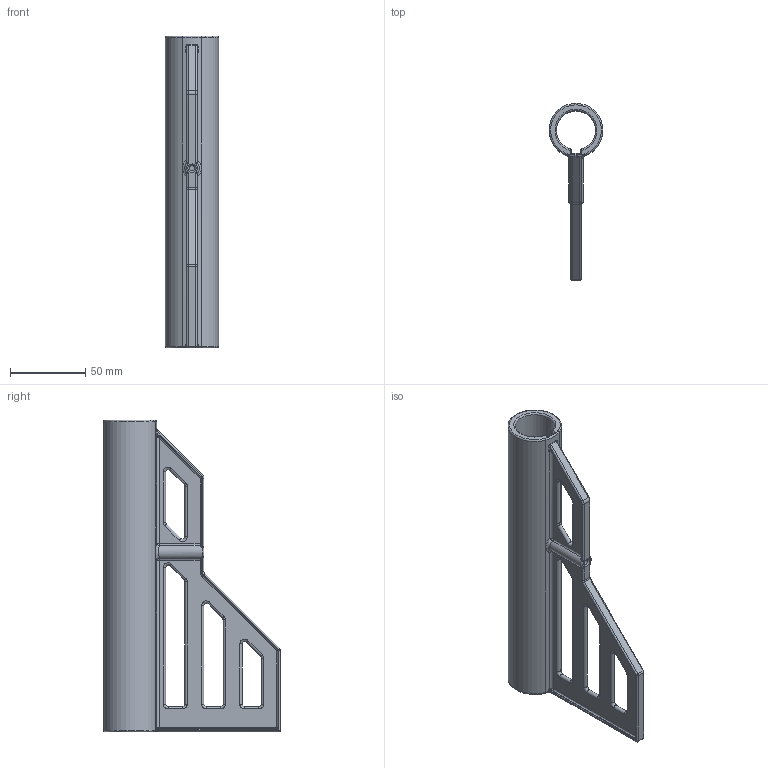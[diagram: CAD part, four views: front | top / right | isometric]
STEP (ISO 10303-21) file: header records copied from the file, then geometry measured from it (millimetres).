
FILE_DESCRIPTION(/* description */ (''),/* implementation_level */ '2;1');
FILE_NAME(/* name */ 'a3bf86a9-df5b-42d4-956c-7e507eac76b7.stp',/* time_stamp */ '2019-04-30T20:53:59-04:00',/* author */ ('suzuki450ltr'),/* organization */ (''),/* preprocessor_version */ 'ST-DEVELOPER v18',/* originating_system */ 'Autodesk Translation Framework v8.2.0.1029',/* authorisation */ '');
FILE_SCHEMA (('AUTOMOTIVE_DESIGN { 1 0 10303 214 3 1 1 }'));
Length unit declared in the file: millimetre
Products named in the file (1): ONE SOLID MODEL Pistol Buffer Tube Stock v4 Copy
Bounding box: 35.67 x 117.5 x 207.38 mm (x, y, z)
Volume: 118447.9 mm3; surface area: 59249.7 mm2
Topology: 1 solids, 1 shells, 236 faces, 576 edges, 331 vertices
Faces by surface type: cylinder 96, bspline 45, torus 45, plane 38, sphere 10, cone 2
Full cylindrical faces by diameter (mm): 3.5 x1
Entity records: 8449 total; most frequent: CARTESIAN_POINT 3026, DIRECTION 1152, ORIENTED_EDGE 1132, EDGE_CURVE 566, AXIS2_PLACEMENT_3D 476, VERTEX_POINT 331, CIRCLE 266, EDGE_LOOP 247
